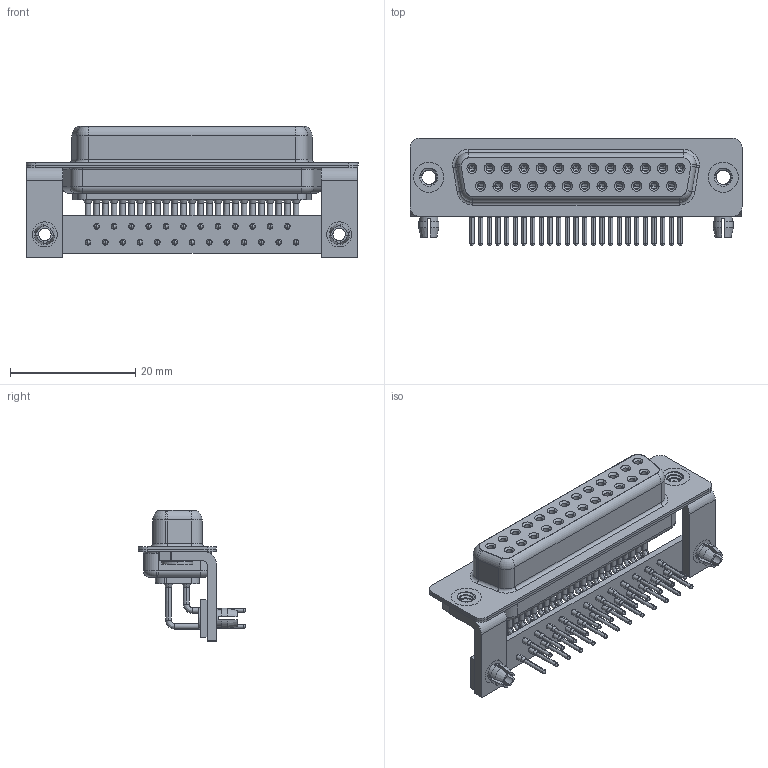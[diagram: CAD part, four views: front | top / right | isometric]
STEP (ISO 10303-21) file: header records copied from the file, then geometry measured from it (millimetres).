
FILE_DESCRIPTION (( 'STEP AP203' ), '1' );
FILE_NAME ('630-M25-340-BN3.STEP', '2018-09-26T01:27:10', ( '' ), ( '' ), 'SwSTEP 2.0', 'SolidWorks 2016', '' );
FILE_SCHEMA (( 'CONFIG_CONTROL_DESIGN' ));
Length unit declared in the file: millimetre
Products named in the file (10): 630-M25-340-BN3; 630M Shell Front_25 Contacts; 630M Shell Rear_25 Contacts; 630M Contact Row 1; 630M Contact Row 2; 630M 4-40 Threaded Rivet_Stabilizer; 630M Stabilizer Bracket; 630M Stabilizer Board_25 Contacts; 630M Board Lock; 630M Housing_25 Contacts
Assembly tree (35 placements, depth 2):
  630-M25-340-BN3
    630M Housing_25 Contacts
    630M Shell Front_25 Contacts
    630M Shell Rear_25 Contacts
    630M Contact Row 1  x13
    630M Contact Row 2  x12
    630M 4-40 Threaded Rivet_Stabilizer  x2
    630M Stabilizer Bracket  x2
    630M Stabilizer Board_25 Contacts
    630M Board Lock  x2
Bounding box: 53.05 x 17.2 x 21 mm (x, y, z)
Volume: 4497.4 mm3; surface area: 11341.9 mm2
Topology: 35 solids, 35 shells, 1796 faces, 4586 edges, 2900 vertices
Faces by surface type: cylinder 816, plane 516, cone 295, bspline 106, torus 63
Entity records: 26597 total; most frequent: CARTESIAN_POINT 5709, DIRECTION 4393, ORIENTED_EDGE 3720, EDGE_CURVE 1860, AXIS2_PLACEMENT_3D 1826, VERTEX_POINT 1191, CIRCLE 1022, EDGE_LOOP 991
